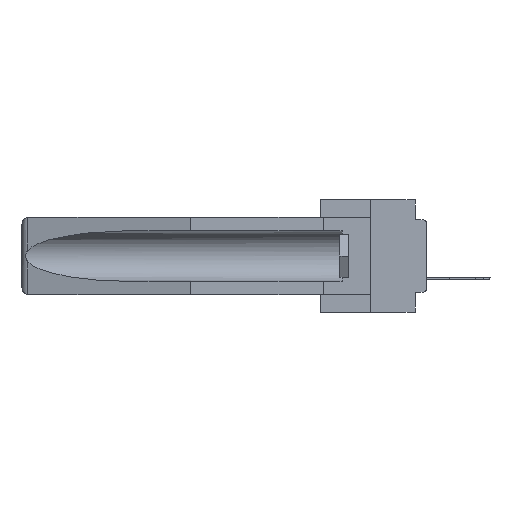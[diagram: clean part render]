
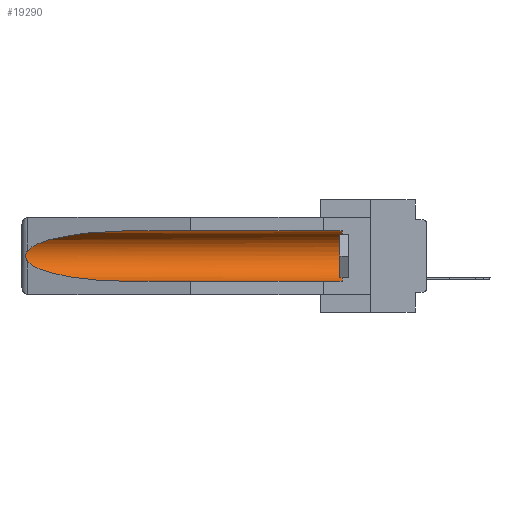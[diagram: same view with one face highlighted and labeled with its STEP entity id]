
A CAD part, left-side view. The second image highlights one B-rep face of the part: STEP entity #19290.
In plain terms, the highlighted cylindrical face has radius 2.857 mm (diameter 5.715 mm), a partial arc.
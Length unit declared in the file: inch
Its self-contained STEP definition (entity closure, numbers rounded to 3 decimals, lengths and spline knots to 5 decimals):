
#796 = CARTESIAN_POINT ( 'NONE',  ( 0.155, 0.126, -0.059 ) ) ;
#942 = AXIS2_PLACEMENT_3D ( 'NONE', #5916, #23767, #1262 ) ;
#1262 = DIRECTION ( 'NONE',  ( 0., 0., 1. ) ) ;
#2459 = CARTESIAN_POINT ( 'NONE',  ( 0.2675, 1.53308, -0.16763 ) ) ;
#2646 = CARTESIAN_POINT ( 'NONE',  ( 0.26654, 1.53092, -0.15636 ) ) ;
#3494 = EDGE_CURVE ( 'NONE', #21751, #14433, #16081, .T. ) ;
#4777 = CARTESIAN_POINT ( 'NONE',  ( 0.26537, 1.52718, -0.14972 ) ) ;
#5394 = VERTEX_POINT ( 'NONE', #27717 ) ;
#5916 = CARTESIAN_POINT ( 'NONE',  ( 0.155, 0.126, -0.1715 ) ) ;
#6222 = EDGE_CURVE ( 'NONE', #5394, #27770, #12567, .T. ) ;
#6516 = EDGE_CURVE ( 'NONE', #14433, #5394, #27127, .T. ) ;
#6986 = CARTESIAN_POINT ( 'NONE',  ( 0.26597, 1.5296, -0.19026 ) ) ;
#7307 = CARTESIAN_POINT ( 'NONE',  ( 0.155, 0.126, -0.284 ) ) ;
#7360 =( BOUNDED_CURVE ( )  B_SPLINE_CURVE ( 3, ( #19451, #14935, #26083, #23830 ),
 .UNSPECIFIED., .F., .F. ) 
 B_SPLINE_CURVE_WITH_KNOTS ( ( 4, 4 ),
 ( 0.1948, 1.5708 ),
 .UNSPECIFIED. ) 
 CURVE ( )  GEOMETRIC_REPRESENTATION_ITEM ( )  RATIONAL_B_SPLINE_CURVE ( ( 1., 0.848, 0.848, 1. ) ) 
 REPRESENTATION_ITEM ( '' )  );
#7534 = LINE ( 'NONE', #19643, #12793 ) ;
#7992 = CARTESIAN_POINT ( 'NONE',  ( 0.155, -0.30754, -0.1715 ) ) ;
#8340 = CARTESIAN_POINT ( 'NONE',  ( 0.155, -0.30754, -0.059 ) ) ;
#8668 = ORIENTED_EDGE ( 'NONE', *, *, #18744, .T. ) ;
#9143 = B_SPLINE_CURVE_WITH_KNOTS ( 'NONE', 3,
 ( #4777, #24860, #2646, #27194, #2459, #18036, #27100, #20369, #6986, #13642 ),
 .UNSPECIFIED., .F., .F.,
 ( 4, 2, 2, 2, 4 ),
 ( 0., 0.00029, 0.00058, 0.00087, 0.00117 ),
 .UNSPECIFIED. ) ;
#9205 = EDGE_CURVE ( 'NONE', #21751, #17529, #7534, .T. ) ;
#9966 = ORIENTED_EDGE ( 'NONE', *, *, #9990, .T. ) ;
#9990 = EDGE_CURVE ( 'NONE', #27770, #11418, #9143, .T. ) ;
#10020 = CYLINDRICAL_SURFACE ( 'NONE', #28555, 0.1125 ) ;
#10891 = CARTESIAN_POINT ( 'NONE',  ( 0.155, 1.07973, -0.059 ) ) ;
#11001 = CARTESIAN_POINT ( 'NONE',  ( 0.26537, 1.52718, -0.14972 ) ) ;
#11418 = VERTEX_POINT ( 'NONE', #12649 ) ;
#12137 = CARTESIAN_POINT ( 'NONE',  ( 0.26537, 1.52718, -0.14972 ) ) ;
#12345 = EDGE_LOOP ( 'NONE', ( #22083, #9966, #8668, #12972, #17643, #12789 ) ) ;
#12567 =( BOUNDED_CURVE ( )  B_SPLINE_CURVE ( 3, ( #10891, #26383, #17582, #11001 ),
 .UNSPECIFIED., .F., .F. ) 
 B_SPLINE_CURVE_WITH_KNOTS ( ( 4, 4 ),
 ( 4.71239, 6.08839 ),
 .UNSPECIFIED. ) 
 CURVE ( )  GEOMETRIC_REPRESENTATION_ITEM ( )  RATIONAL_B_SPLINE_CURVE ( ( 1., 0.848, 0.848, 1. ) ) 
 REPRESENTATION_ITEM ( '' )  );
#12649 = CARTESIAN_POINT ( 'NONE',  ( 0.26537, 1.52718, -0.19328 ) ) ;
#12789 = ORIENTED_EDGE ( 'NONE', *, *, #6516, .T. ) ;
#12793 = VECTOR ( 'NONE', #15324, 39.37008 ) ;
#12972 = ORIENTED_EDGE ( 'NONE', *, *, #9205, .F. ) ;
#13642 = CARTESIAN_POINT ( 'NONE',  ( 0.26537, 1.52718, -0.19328 ) ) ;
#14433 = VERTEX_POINT ( 'NONE', #796 ) ;
#14935 = CARTESIAN_POINT ( 'NONE',  ( 0.25451, 1.48313, -0.24835 ) ) ;
#15324 = DIRECTION ( 'NONE',  ( 0., 1., 0. ) ) ;
#15450 = DIRECTION ( 'NONE',  ( 0., 1., 0. ) ) ;
#15931 = FACE_OUTER_BOUND ( 'NONE', #12345, .T. ) ;
#16081 = CIRCLE ( 'NONE', #942, 0.1125 ) ;
#16957 = CARTESIAN_POINT ( 'NONE',  ( 0.155, 1.07973, -0.284 ) ) ;
#17152 = DIRECTION ( 'NONE',  ( 0., 1., 0. ) ) ;
#17529 = VERTEX_POINT ( 'NONE', #16957 ) ;
#17582 = CARTESIAN_POINT ( 'NONE',  ( 0.25451, 1.48313, -0.09465 ) ) ;
#17643 = ORIENTED_EDGE ( 'NONE', *, *, #3494, .T. ) ;
#18036 = CARTESIAN_POINT ( 'NONE',  ( 0.2675, 1.53308, -0.17534 ) ) ;
#18744 = EDGE_CURVE ( 'NONE', #11418, #17529, #7360, .T. ) ;
#19290 = ADVANCED_FACE ( 'NONE', ( #15931 ), #10020, .F. ) ;
#19451 = CARTESIAN_POINT ( 'NONE',  ( 0.26537, 1.52718, -0.19328 ) ) ;
#19643 = CARTESIAN_POINT ( 'NONE',  ( 0.155, -0.30754, -0.284 ) ) ;
#20369 = CARTESIAN_POINT ( 'NONE',  ( 0.26655, 1.53094, -0.18657 ) ) ;
#21751 = VERTEX_POINT ( 'NONE', #7307 ) ;
#22083 = ORIENTED_EDGE ( 'NONE', *, *, #6222, .T. ) ;
#23767 = DIRECTION ( 'NONE',  ( 0., -1., 0. ) ) ;
#23830 = CARTESIAN_POINT ( 'NONE',  ( 0.155, 1.07973, -0.284 ) ) ;
#24860 = CARTESIAN_POINT ( 'NONE',  ( 0.26597, 1.52961, -0.15275 ) ) ;
#25767 = DIRECTION ( 'NONE',  ( 0., 0., 1. ) ) ;
#26083 = CARTESIAN_POINT ( 'NONE',  ( 0.21114, 1.30732, -0.284 ) ) ;
#26383 = CARTESIAN_POINT ( 'NONE',  ( 0.21114, 1.30732, -0.059 ) ) ;
#26440 = VECTOR ( 'NONE', #15450, 39.37008 ) ;
#27100 = CARTESIAN_POINT ( 'NONE',  ( 0.2673, 1.53269, -0.17917 ) ) ;
#27127 = LINE ( 'NONE', #8340, #26440 ) ;
#27194 = CARTESIAN_POINT ( 'NONE',  ( 0.2673, 1.5327, -0.16383 ) ) ;
#27717 = CARTESIAN_POINT ( 'NONE',  ( 0.155, 1.07973, -0.059 ) ) ;
#27770 = VERTEX_POINT ( 'NONE', #12137 ) ;
#28555 = AXIS2_PLACEMENT_3D ( 'NONE', #7992, #17152, #25767 ) ;
